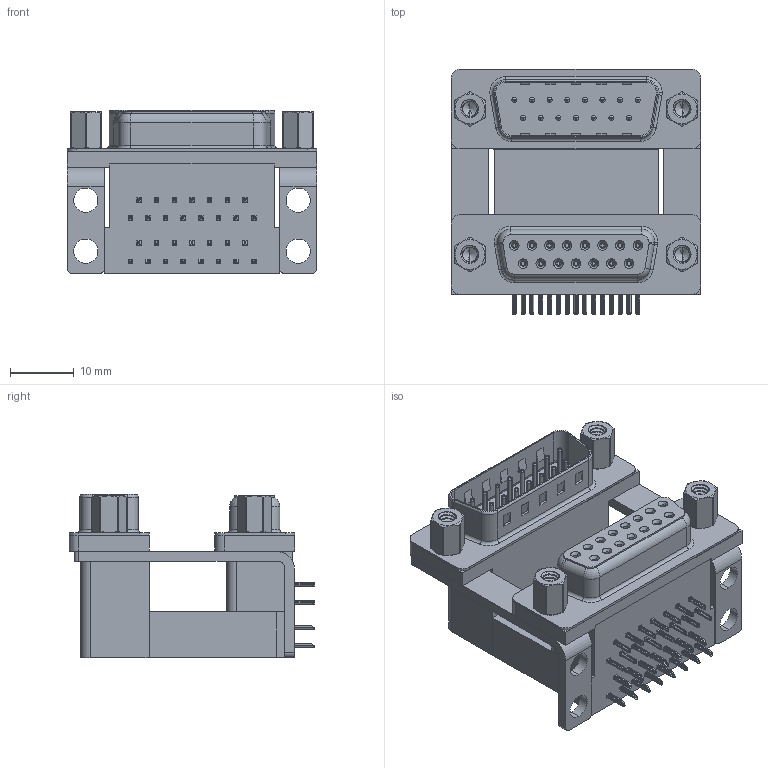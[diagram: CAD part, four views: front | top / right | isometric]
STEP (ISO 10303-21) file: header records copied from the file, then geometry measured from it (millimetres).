
FILE_DESCRIPTION (( 'STEP AP203' ), '1' );
FILE_NAME ('663-015-264-009.STEP', '2022-06-17T22:51:07', ( '' ), ( '' ), 'SwSTEP 2.0', 'SolidWorks 2020', '' );
FILE_SCHEMA (( 'CONFIG_CONTROL_DESIGN' ));
Length unit declared in the file: millimetre
Products named in the file (13): 663 Threaded Rivet_4-40; 663 Contact Top Lower; 663 Mounting Bracket_NoneH; 663 Housing Spacer_15 Contacts H; 663 Housing Lower_15 Contacts; 663 4-40 Hex Standoff 5; 663 Housing Upper_15 Contacts H; 663 Contact Bottom Upper_H; 663 Shell Receptacle_15 Contacts; 663 Contact Top Upper_H; 663 Shell Plug_15 Contacts; 663 Contact Bottom Lower; 663-015-264-009
Assembly tree (45 placements, depth 2):
  663-015-264-009
    663 Housing Lower_15 Contacts
    663 Housing Spacer_15 Contacts H
    663 Housing Upper_15 Contacts H
    663 Shell Receptacle_15 Contacts
    663 Shell Plug_15 Contacts
    663 Contact Bottom Lower  x7
    663 Contact Top Lower  x8
    663 Contact Bottom Upper_H  x7
    663 Contact Top Upper_H  x8
    663 Mounting Bracket_NoneH  x2
    663 Threaded Rivet_4-40  x4
    663 4-40 Hex Standoff 5  x4
Bounding box: 39.19 x 38.59 x 25.6 mm (x, y, z)
Volume: 16404.3 mm3; surface area: 18372.5 mm2
Topology: 45 solids, 45 shells, 4164 faces, 10739 edges, 6729 vertices
Faces by surface type: plane 2059, cylinder 1158, bspline 548, cone 240, torus 159
Entity records: 48680 total; most frequent: CARTESIAN_POINT 15127, ORIENTED_EDGE 6618, DIRECTION 6186, EDGE_CURVE 3309, VECTOR 2198, LINE 2198, VERTEX_POINT 2115, AXIS2_PLACEMENT_3D 1994
